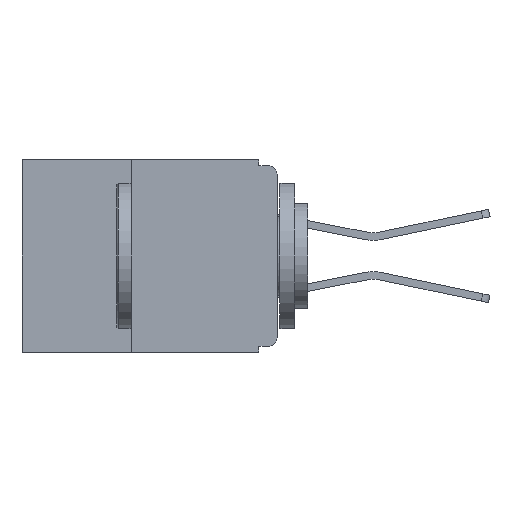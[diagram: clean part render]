
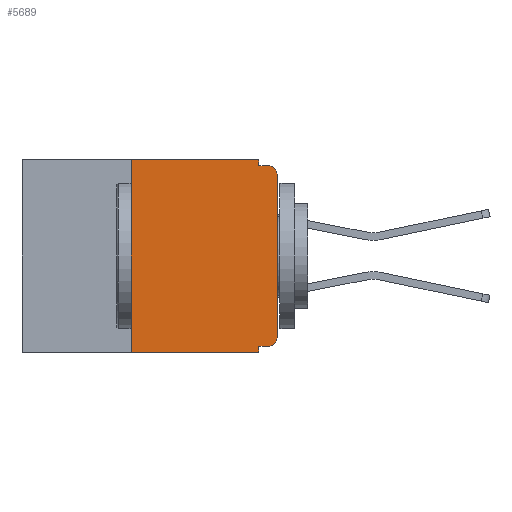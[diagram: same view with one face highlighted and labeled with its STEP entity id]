
A CAD part, left-side view. The second image highlights one B-rep face of the part: STEP entity #5689.
In plain terms, the highlighted planar face has unit normal (-1, 0, 0).
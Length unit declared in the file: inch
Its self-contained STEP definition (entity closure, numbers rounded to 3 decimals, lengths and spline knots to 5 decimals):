
#126 = CARTESIAN_POINT ( 'NONE',  ( 0., 0.25, -0.33 ) ) ;
#239 = ORIENTED_EDGE ( 'NONE', *, *, #18440, .T. ) ;
#274 = LINE ( 'NONE', #11648, #19635 ) ;
#314 = VERTEX_POINT ( 'NONE', #1608 ) ;
#708 = CARTESIAN_POINT ( 'NONE',  ( 0., 0.015, -0.305 ) ) ;
#1165 = VERTEX_POINT ( 'NONE', #20655 ) ;
#1321 = CARTESIAN_POINT ( 'NONE',  ( 0., 0.015, -0.025 ) ) ;
#1608 = CARTESIAN_POINT ( 'NONE',  ( 0., 0.015, -0.32 ) ) ;
#1613 = VERTEX_POINT ( 'NONE', #6653 ) ;
#1694 = DIRECTION ( 'NONE',  ( 0., 0., -1. ) ) ;
#3192 = DIRECTION ( 'NONE',  ( 0., 0., -1. ) ) ;
#3460 = EDGE_CURVE ( 'NONE', #4710, #1165, #19132, .T. ) ;
#4110 = EDGE_CURVE ( 'NONE', #17619, #20181, #23004, .T. ) ;
#4623 = CARTESIAN_POINT ( 'NONE',  ( 0., 0., -0.305 ) ) ;
#4710 = VERTEX_POINT ( 'NONE', #12210 ) ;
#4724 = EDGE_CURVE ( 'NONE', #9496, #1165, #274, .T. ) ;
#5048 = DIRECTION ( 'NONE',  ( 0., 0., -1. ) ) ;
#5608 = CARTESIAN_POINT ( 'NONE',  ( 0., 0.031, -0.33 ) ) ;
#5689 = ADVANCED_FACE ( 'NONE', ( #14872 ), #7384, .F. ) ;
#5798 = ORIENTED_EDGE ( 'NONE', *, *, #10909, .T. ) ;
#5818 = CARTESIAN_POINT ( 'NONE',  ( 0., 0., -0.32 ) ) ;
#5964 = EDGE_CURVE ( 'NONE', #9496, #1613, #18337, .T. ) ;
#6653 = CARTESIAN_POINT ( 'NONE',  ( 0., 0.25, 0. ) ) ;
#6798 = DIRECTION ( 'NONE',  ( 0., -1., 0. ) ) ;
#6907 = DIRECTION ( 'NONE',  ( 0., 0., -1. ) ) ;
#6908 = DIRECTION ( 'NONE',  ( 1., 0., 0. ) ) ;
#7204 = CARTESIAN_POINT ( 'NONE',  ( 0., 0.437, 0. ) ) ;
#7248 = EDGE_CURVE ( 'NONE', #12051, #17619, #17662, .T. ) ;
#7384 = PLANE ( 'NONE',  #14532 ) ;
#7632 = ORIENTED_EDGE ( 'NONE', *, *, #5964, .F. ) ;
#8886 = CARTESIAN_POINT ( 'NONE',  ( 0., 0., 0. ) ) ;
#9163 = EDGE_CURVE ( 'NONE', #18979, #12808, #20756, .T. ) ;
#9318 = AXIS2_PLACEMENT_3D ( 'NONE', #1321, #14510, #3192 ) ;
#9496 = VERTEX_POINT ( 'NONE', #13775 ) ;
#9695 = EDGE_CURVE ( 'NONE', #1613, #12051, #23171, .T. ) ;
#10583 = ORIENTED_EDGE ( 'NONE', *, *, #23216, .F. ) ;
#10777 = DIRECTION ( 'NONE',  ( 0., 0., 1. ) ) ;
#10909 = EDGE_CURVE ( 'NONE', #314, #18979, #14075, .T. ) ;
#11096 = AXIS2_PLACEMENT_3D ( 'NONE', #708, #12991, #1694 ) ;
#11465 = ORIENTED_EDGE ( 'NONE', *, *, #9695, .F. ) ;
#11648 = CARTESIAN_POINT ( 'NONE',  ( 0., 0.437, -0.33 ) ) ;
#11784 = DIRECTION ( 'NONE',  ( 0., -1., 0. ) ) ;
#11825 = DIRECTION ( 'NONE',  ( 0., -1., 0. ) ) ;
#11848 = CARTESIAN_POINT ( 'NONE',  ( 0., 0., -0.01 ) ) ;
#12051 = VERTEX_POINT ( 'NONE', #18377 ) ;
#12210 = CARTESIAN_POINT ( 'NONE',  ( 0., 0.031, -0.32 ) ) ;
#12761 = VECTOR ( 'NONE', #15602, 39.37008 ) ;
#12808 = VERTEX_POINT ( 'NONE', #20664 ) ;
#12991 = DIRECTION ( 'NONE',  ( -1., 0., 0. ) ) ;
#13350 = CIRCLE ( 'NONE', #9318, 0.015 ) ;
#13775 = CARTESIAN_POINT ( 'NONE',  ( 0., 0.25, -0.33 ) ) ;
#14075 = CIRCLE ( 'NONE', #11096, 0.015 ) ;
#14510 = DIRECTION ( 'NONE',  ( -1., 0., 0. ) ) ;
#14532 = AXIS2_PLACEMENT_3D ( 'NONE', #7204, #6908, #6907 ) ;
#14872 = FACE_OUTER_BOUND ( 'NONE', #23154, .T. ) ;
#15602 = DIRECTION ( 'NONE',  ( 0., 0., -1. ) ) ;
#15807 = CARTESIAN_POINT ( 'NONE',  ( 0., 0.031, 0. ) ) ;
#15846 = VECTOR ( 'NONE', #10777, 39.37008 ) ;
#15868 = ORIENTED_EDGE ( 'NONE', *, *, #7248, .F. ) ;
#17619 = VERTEX_POINT ( 'NONE', #19512 ) ;
#17662 = LINE ( 'NONE', #15807, #12761 ) ;
#18337 = LINE ( 'NONE', #126, #23084 ) ;
#18377 = CARTESIAN_POINT ( 'NONE',  ( 0., 0.031, 0. ) ) ;
#18434 = VECTOR ( 'NONE', #6798, 39.37008 ) ;
#18440 = EDGE_CURVE ( 'NONE', #12808, #20181, #13350, .T. ) ;
#18570 = VECTOR ( 'NONE', #5048, 39.37008 ) ;
#18954 = DIRECTION ( 'NONE',  ( 0., 1., 0. ) ) ;
#18979 = VERTEX_POINT ( 'NONE', #4623 ) ;
#19132 = LINE ( 'NONE', #5608, #18570 ) ;
#19334 = ORIENTED_EDGE ( 'NONE', *, *, #3460, .F. ) ;
#19512 = CARTESIAN_POINT ( 'NONE',  ( 0., 0.031, -0.01 ) ) ;
#19635 = VECTOR ( 'NONE', #11784, 39.37008 ) ;
#20181 = VERTEX_POINT ( 'NONE', #21070 ) ;
#20201 = ORIENTED_EDGE ( 'NONE', *, *, #4110, .F. ) ;
#20655 = CARTESIAN_POINT ( 'NONE',  ( 0., 0.031, -0.33 ) ) ;
#20664 = CARTESIAN_POINT ( 'NONE',  ( 0., 0., -0.025 ) ) ;
#20756 = LINE ( 'NONE', #8886, #15846 ) ;
#21070 = CARTESIAN_POINT ( 'NONE',  ( 0., 0.015, -0.01 ) ) ;
#21612 = CARTESIAN_POINT ( 'NONE',  ( 0., 0.437, 0. ) ) ;
#22458 = VECTOR ( 'NONE', #11825, 39.37008 ) ;
#22552 = LINE ( 'NONE', #5818, #23098 ) ;
#23004 = LINE ( 'NONE', #11848, #22458 ) ;
#23084 = VECTOR ( 'NONE', #23890, 39.37008 ) ;
#23098 = VECTOR ( 'NONE', #18954, 39.37008 ) ;
#23154 = EDGE_LOOP ( 'NONE', ( #23218, #239, #20201, #15868, #11465, #7632, #23501, #19334, #10583, #5798 ) ) ;
#23171 = LINE ( 'NONE', #21612, #18434 ) ;
#23216 = EDGE_CURVE ( 'NONE', #314, #4710, #22552, .T. ) ;
#23218 = ORIENTED_EDGE ( 'NONE', *, *, #9163, .T. ) ;
#23501 = ORIENTED_EDGE ( 'NONE', *, *, #4724, .T. ) ;
#23890 = DIRECTION ( 'NONE',  ( 0., 0., 1. ) ) ;
